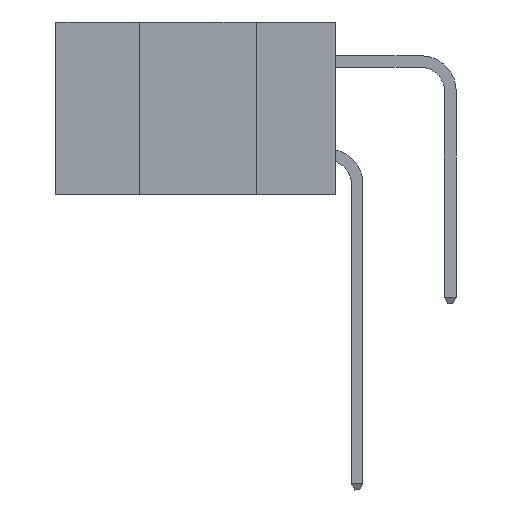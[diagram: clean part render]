
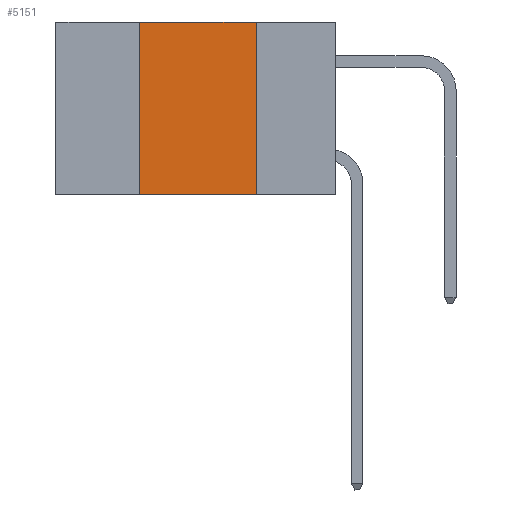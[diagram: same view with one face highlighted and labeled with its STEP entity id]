
A CAD part, left-side view. The second image highlights one B-rep face of the part: STEP entity #5151.
In plain terms, the highlighted planar face has unit normal (-1, 0, 0).
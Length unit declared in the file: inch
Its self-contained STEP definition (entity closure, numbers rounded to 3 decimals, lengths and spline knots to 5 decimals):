
#955 = CARTESIAN_POINT ( 'NONE',  ( 0., 0.42, -0.37 ) ) ;
#1318 = LINE ( 'NONE', #2274, #23202 ) ;
#1832 = ORIENTED_EDGE ( 'NONE', *, *, #13076, .F. ) ;
#1918 = VECTOR ( 'NONE', #10136, 39.37008 ) ;
#2274 = CARTESIAN_POINT ( 'NONE',  ( 0., 0.6, -0.37 ) ) ;
#4795 = DIRECTION ( 'NONE',  ( 0., 0., 1. ) ) ;
#5151 = ADVANCED_FACE ( 'NONE', ( #10615 ), #17766, .F. ) ;
#5937 = AXIS2_PLACEMENT_3D ( 'NONE', #19509, #13197, #19972 ) ;
#6758 = EDGE_CURVE ( 'NONE', #8853, #13608, #1318, .T. ) ;
#6864 = CARTESIAN_POINT ( 'NONE',  ( 0., 0.42, 0. ) ) ;
#7112 = VECTOR ( 'NONE', #4795, 39.37008 ) ;
#7145 = ORIENTED_EDGE ( 'NONE', *, *, #18159, .F. ) ;
#7615 = LINE ( 'NONE', #18505, #1918 ) ;
#8238 = VERTEX_POINT ( 'NONE', #21278 ) ;
#8853 = VERTEX_POINT ( 'NONE', #955 ) ;
#9239 = VECTOR ( 'NONE', #23502, 39.37008 ) ;
#9758 = EDGE_CURVE ( 'NONE', #8853, #8238, #14363, .T. ) ;
#10136 = DIRECTION ( 'NONE',  ( 0., 0., -1. ) ) ;
#10615 = FACE_OUTER_BOUND ( 'NONE', #24134, .T. ) ;
#10705 = CARTESIAN_POINT ( 'NONE',  ( 0., 0.6, 0. ) ) ;
#12204 = CARTESIAN_POINT ( 'NONE',  ( 0., 0.17, 0. ) ) ;
#13076 = EDGE_CURVE ( 'NONE', #8238, #19825, #26506, .T. ) ;
#13197 = DIRECTION ( 'NONE',  ( 1., 0., 0. ) ) ;
#13608 = VERTEX_POINT ( 'NONE', #22255 ) ;
#14363 = LINE ( 'NONE', #6864, #7112 ) ;
#17766 = PLANE ( 'NONE',  #5937 ) ;
#18159 = EDGE_CURVE ( 'NONE', #19825, #13608, #7615, .T. ) ;
#18505 = CARTESIAN_POINT ( 'NONE',  ( 0., 0.17, 0. ) ) ;
#19509 = CARTESIAN_POINT ( 'NONE',  ( 0., 0.6, 0. ) ) ;
#19825 = VERTEX_POINT ( 'NONE', #12204 ) ;
#19972 = DIRECTION ( 'NONE',  ( 0., 0., -1. ) ) ;
#21249 = ORIENTED_EDGE ( 'NONE', *, *, #6758, .T. ) ;
#21278 = CARTESIAN_POINT ( 'NONE',  ( 0., 0.42, 0. ) ) ;
#22255 = CARTESIAN_POINT ( 'NONE',  ( 0., 0.17, -0.37 ) ) ;
#23202 = VECTOR ( 'NONE', #24256, 39.37008 ) ;
#23502 = DIRECTION ( 'NONE',  ( 0., -1., 0. ) ) ;
#24134 = EDGE_LOOP ( 'NONE', ( #7145, #1832, #25328, #21249 ) ) ;
#24256 = DIRECTION ( 'NONE',  ( 0., -1., 0. ) ) ;
#25328 = ORIENTED_EDGE ( 'NONE', *, *, #9758, .F. ) ;
#26506 = LINE ( 'NONE', #10705, #9239 ) ;
